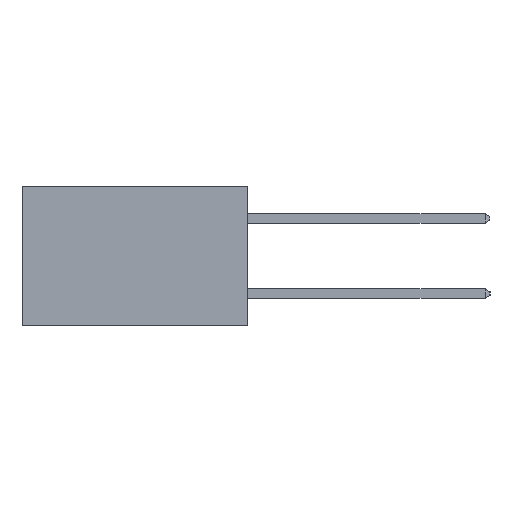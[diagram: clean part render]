
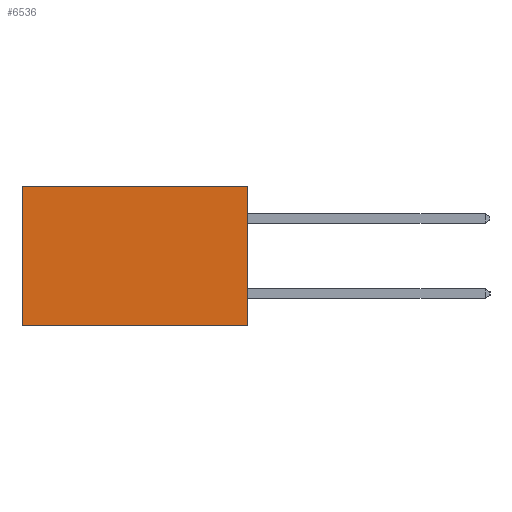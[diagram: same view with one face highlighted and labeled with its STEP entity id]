
A CAD part, left-side view. The second image highlights one B-rep face of the part: STEP entity #6536.
In plain terms, the highlighted planar face has unit normal (-1, 0, 0).
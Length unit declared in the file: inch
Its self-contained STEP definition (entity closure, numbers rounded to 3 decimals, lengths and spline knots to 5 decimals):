
#95 = LINE ( 'NONE', #9262, #12142 ) ;
#604 = AXIS2_PLACEMENT_3D ( 'NONE', #5501, #5453, #5451 ) ;
#681 = CARTESIAN_POINT ( 'NONE',  ( 0.2615, 0., -0.37 ) ) ;
#880 = CARTESIAN_POINT ( 'NONE',  ( 0.2615, 0., 0. ) ) ;
#1268 = DIRECTION ( 'NONE',  ( 0., 1., 0. ) ) ;
#1827 = VECTOR ( 'NONE', #1268, 39.37008 ) ;
#1868 = DIRECTION ( 'NONE',  ( 0., 1., 0. ) ) ;
#2502 = EDGE_CURVE ( 'NONE', #9229, #11621, #95, .T. ) ;
#3181 = VECTOR ( 'NONE', #7682, 39.37008 ) ;
#4738 = CARTESIAN_POINT ( 'NONE',  ( 0.2615, 0.6, -0.37 ) ) ;
#5451 = DIRECTION ( 'NONE',  ( 0., 0., -1. ) ) ;
#5453 = DIRECTION ( 'NONE',  ( 1., 0., 0. ) ) ;
#5501 = CARTESIAN_POINT ( 'NONE',  ( 0.2615, 0., -0.37 ) ) ;
#5505 = PLANE ( 'NONE',  #604 ) ;
#5820 = ORIENTED_EDGE ( 'NONE', *, *, #10483, .T. ) ;
#6021 = ORIENTED_EDGE ( 'NONE', *, *, #13581, .F. ) ;
#6220 = LINE ( 'NONE', #13433, #3181 ) ;
#6536 = ADVANCED_FACE ( 'NONE', ( #8970 ), #5505, .F. ) ;
#6574 = ORIENTED_EDGE ( 'NONE', *, *, #8087, .T. ) ;
#6849 = DIRECTION ( 'NONE',  ( 0., 0., -1. ) ) ;
#7138 = EDGE_LOOP ( 'NONE', ( #5820, #6021, #9597, #6574 ) ) ;
#7421 = VERTEX_POINT ( 'NONE', #14130 ) ;
#7682 = DIRECTION ( 'NONE',  ( 0., 0., -1. ) ) ;
#7724 = CARTESIAN_POINT ( 'NONE',  ( 0.2615, 0., 0. ) ) ;
#8087 = EDGE_CURVE ( 'NONE', #9229, #7421, #11132, .T. ) ;
#8970 = FACE_OUTER_BOUND ( 'NONE', #7138, .T. ) ;
#9229 = VERTEX_POINT ( 'NONE', #7724 ) ;
#9262 = CARTESIAN_POINT ( 'NONE',  ( 0.2615, 0., -0.37 ) ) ;
#9597 = ORIENTED_EDGE ( 'NONE', *, *, #2502, .F. ) ;
#9679 = VERTEX_POINT ( 'NONE', #4738 ) ;
#10483 = EDGE_CURVE ( 'NONE', #7421, #9679, #6220, .T. ) ;
#10802 = CARTESIAN_POINT ( 'NONE',  ( 0.2615, 0., -0.37 ) ) ;
#11132 = LINE ( 'NONE', #880, #1827 ) ;
#11621 = VERTEX_POINT ( 'NONE', #10802 ) ;
#12142 = VECTOR ( 'NONE', #6849, 39.37008 ) ;
#13433 = CARTESIAN_POINT ( 'NONE',  ( 0.2615, 0.6, -0.37 ) ) ;
#13581 = EDGE_CURVE ( 'NONE', #11621, #9679, #14572, .T. ) ;
#14130 = CARTESIAN_POINT ( 'NONE',  ( 0.2615, 0.6, 0. ) ) ;
#14230 = VECTOR ( 'NONE', #1868, 39.37008 ) ;
#14572 = LINE ( 'NONE', #681, #14230 ) ;
